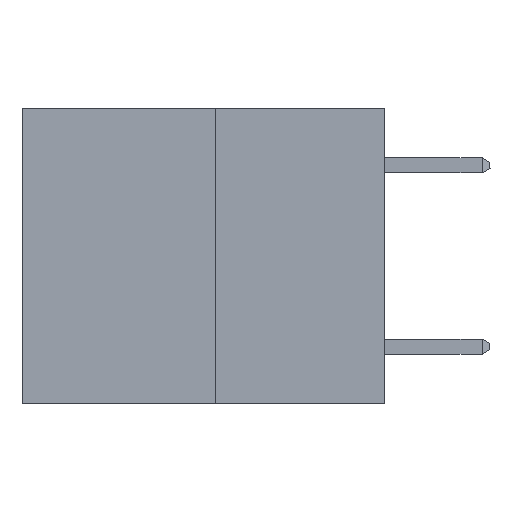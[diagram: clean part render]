
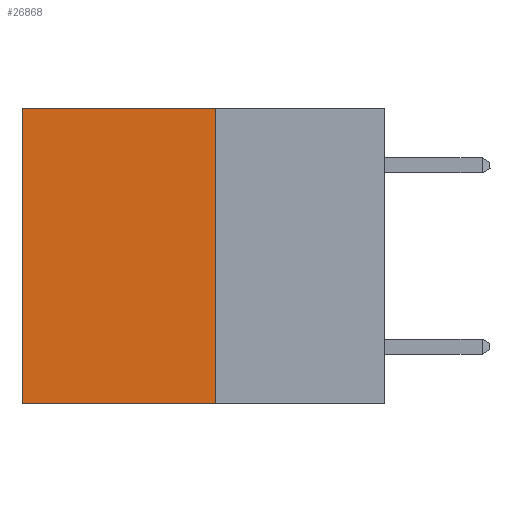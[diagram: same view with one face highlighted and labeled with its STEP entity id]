
A CAD part, left-side view. The second image highlights one B-rep face of the part: STEP entity #26868.
In plain terms, the highlighted planar face has unit normal (-1, 0, 0).
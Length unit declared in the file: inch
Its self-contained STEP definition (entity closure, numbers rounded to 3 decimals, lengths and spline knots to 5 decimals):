
#664 = CARTESIAN_POINT ( 'NONE',  ( 0.3165, 0.28, 0. ) ) ;
#2090 = DIRECTION ( 'NONE',  ( 0., 0., -1. ) ) ;
#2644 = ORIENTED_EDGE ( 'NONE', *, *, #6487, .T. ) ;
#3193 = DIRECTION ( 'NONE',  ( 0., 1., 0. ) ) ;
#5584 = LINE ( 'NONE', #9426, #15885 ) ;
#5801 = FACE_OUTER_BOUND ( 'NONE', #7563, .T. ) ;
#6184 = CARTESIAN_POINT ( 'NONE',  ( 0.3165, 0.28, -0.49 ) ) ;
#6487 = EDGE_CURVE ( 'NONE', #14102, #23934, #22630, .T. ) ;
#6617 = DIRECTION ( 'NONE',  ( 0., 1., 0. ) ) ;
#7563 = EDGE_LOOP ( 'NONE', ( #9110, #17043, #24073, #2644 ) ) ;
#8257 = CARTESIAN_POINT ( 'NONE',  ( 0.3165, 0.6, -0.49 ) ) ;
#9110 = ORIENTED_EDGE ( 'NONE', *, *, #19743, .T. ) ;
#9179 = VECTOR ( 'NONE', #2090, 39.37008 ) ;
#9426 = CARTESIAN_POINT ( 'NONE',  ( 0.3165, 0.28, -0.49 ) ) ;
#9455 = EDGE_CURVE ( 'NONE', #14102, #11538, #5584, .T. ) ;
#10705 = VECTOR ( 'NONE', #6617, 39.37008 ) ;
#11032 = CARTESIAN_POINT ( 'NONE',  ( 0.3165, 0.28, -0.49 ) ) ;
#11376 = DIRECTION ( 'NONE',  ( 0., 0., -1. ) ) ;
#11538 = VERTEX_POINT ( 'NONE', #6184 ) ;
#12412 = CARTESIAN_POINT ( 'NONE',  ( 0.3165, 0.6, -0.49 ) ) ;
#12469 = EDGE_CURVE ( 'NONE', #11538, #14335, #22972, .T. ) ;
#12836 = CARTESIAN_POINT ( 'NONE',  ( 0.3165, 0.28, 0. ) ) ;
#13435 = CARTESIAN_POINT ( 'NONE',  ( 0.3165, 0.6, 0. ) ) ;
#14102 = VERTEX_POINT ( 'NONE', #664 ) ;
#14303 = DIRECTION ( 'NONE',  ( 1., 0., 0. ) ) ;
#14335 = VERTEX_POINT ( 'NONE', #12412 ) ;
#14372 = VECTOR ( 'NONE', #3193, 39.37008 ) ;
#15885 = VECTOR ( 'NONE', #11376, 39.37008 ) ;
#16678 = CARTESIAN_POINT ( 'NONE',  ( 0.3165, 0.28, -0.49 ) ) ;
#17043 = ORIENTED_EDGE ( 'NONE', *, *, #12469, .F. ) ;
#18401 = PLANE ( 'NONE',  #25507 ) ;
#19743 = EDGE_CURVE ( 'NONE', #23934, #14335, #24440, .T. ) ;
#22630 = LINE ( 'NONE', #12836, #10705 ) ;
#22972 = LINE ( 'NONE', #11032, #14372 ) ;
#23934 = VERTEX_POINT ( 'NONE', #13435 ) ;
#24073 = ORIENTED_EDGE ( 'NONE', *, *, #9455, .F. ) ;
#24440 = LINE ( 'NONE', #8257, #9179 ) ;
#25055 = DIRECTION ( 'NONE',  ( 0., 0., -1. ) ) ;
#25507 = AXIS2_PLACEMENT_3D ( 'NONE', #16678, #14303, #25055 ) ;
#26868 = ADVANCED_FACE ( 'NONE', ( #5801 ), #18401, .F. ) ;
